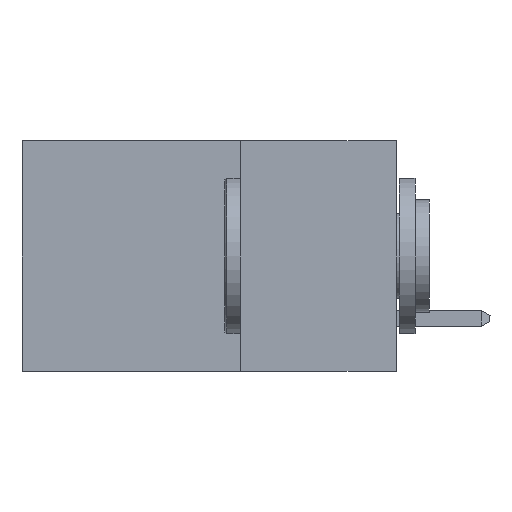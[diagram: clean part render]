
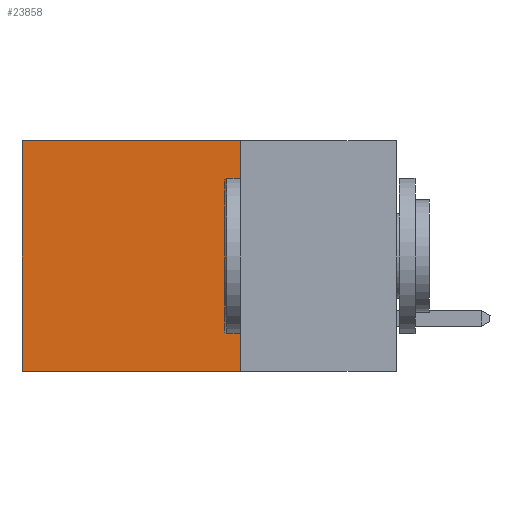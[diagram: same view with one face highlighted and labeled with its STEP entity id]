
A CAD part, left-side view. The second image highlights one B-rep face of the part: STEP entity #23858.
In plain terms, the highlighted planar face has unit normal (-1, 0, 0).
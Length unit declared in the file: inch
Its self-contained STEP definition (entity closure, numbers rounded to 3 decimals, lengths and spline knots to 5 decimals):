
#175 = CARTESIAN_POINT ( 'NONE',  ( 0.2615, 0.6, -0.37 ) ) ;
#2662 = ORIENTED_EDGE ( 'NONE', *, *, #12670, .T. ) ;
#3782 = CARTESIAN_POINT ( 'NONE',  ( 0.2615, 0.6, 0. ) ) ;
#4053 = VECTOR ( 'NONE', #20506, 39.37008 ) ;
#4208 = LINE ( 'NONE', #9891, #14523 ) ;
#4906 = EDGE_CURVE ( 'NONE', #19421, #7108, #15050, .T. ) ;
#5572 = LINE ( 'NONE', #8794, #8215 ) ;
#5892 = AXIS2_PLACEMENT_3D ( 'NONE', #9413, #20154, #14471 ) ;
#5953 = ORIENTED_EDGE ( 'NONE', *, *, #4906, .F. ) ;
#6302 = CARTESIAN_POINT ( 'NONE',  ( 0.2615, 0.25, 0. ) ) ;
#6476 = LINE ( 'NONE', #19568, #10909 ) ;
#7108 = VERTEX_POINT ( 'NONE', #175 ) ;
#8215 = VECTOR ( 'NONE', #14837, 39.37008 ) ;
#8794 = CARTESIAN_POINT ( 'NONE',  ( 0.2615, 0.25, 0. ) ) ;
#9413 = CARTESIAN_POINT ( 'NONE',  ( 0.2615, 0.25, -0.37 ) ) ;
#9891 = CARTESIAN_POINT ( 'NONE',  ( 0.2615, 0.25, -0.37 ) ) ;
#10721 = EDGE_LOOP ( 'NONE', ( #11430, #5953, #19419, #2662 ) ) ;
#10909 = VECTOR ( 'NONE', #21679, 39.37008 ) ;
#10969 = EDGE_CURVE ( 'NONE', #23068, #7108, #6476, .T. ) ;
#11430 = ORIENTED_EDGE ( 'NONE', *, *, #10969, .T. ) ;
#12670 = EDGE_CURVE ( 'NONE', #24289, #23068, #5572, .T. ) ;
#13083 = CARTESIAN_POINT ( 'NONE',  ( 0.2615, 0.25, -0.37 ) ) ;
#13115 = CARTESIAN_POINT ( 'NONE',  ( 0.2615, 0.25, -0.37 ) ) ;
#14471 = DIRECTION ( 'NONE',  ( 0., 0., -1. ) ) ;
#14523 = VECTOR ( 'NONE', #16927, 39.37008 ) ;
#14837 = DIRECTION ( 'NONE',  ( 0., 1., 0. ) ) ;
#15050 = LINE ( 'NONE', #13083, #4053 ) ;
#16927 = DIRECTION ( 'NONE',  ( 0., 0., -1. ) ) ;
#18419 = PLANE ( 'NONE',  #5892 ) ;
#19419 = ORIENTED_EDGE ( 'NONE', *, *, #22739, .F. ) ;
#19421 = VERTEX_POINT ( 'NONE', #13115 ) ;
#19568 = CARTESIAN_POINT ( 'NONE',  ( 0.2615, 0.6, -0.37 ) ) ;
#20154 = DIRECTION ( 'NONE',  ( 1., 0., 0. ) ) ;
#20506 = DIRECTION ( 'NONE',  ( 0., 1., 0. ) ) ;
#21679 = DIRECTION ( 'NONE',  ( 0., 0., -1. ) ) ;
#22739 = EDGE_CURVE ( 'NONE', #24289, #19421, #4208, .T. ) ;
#23068 = VERTEX_POINT ( 'NONE', #3782 ) ;
#23858 = ADVANCED_FACE ( 'NONE', ( #24374 ), #18419, .F. ) ;
#24289 = VERTEX_POINT ( 'NONE', #6302 ) ;
#24374 = FACE_OUTER_BOUND ( 'NONE', #10721, .T. ) ;
